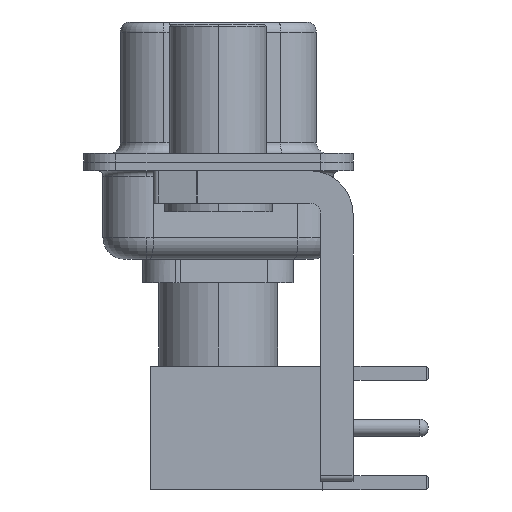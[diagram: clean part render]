
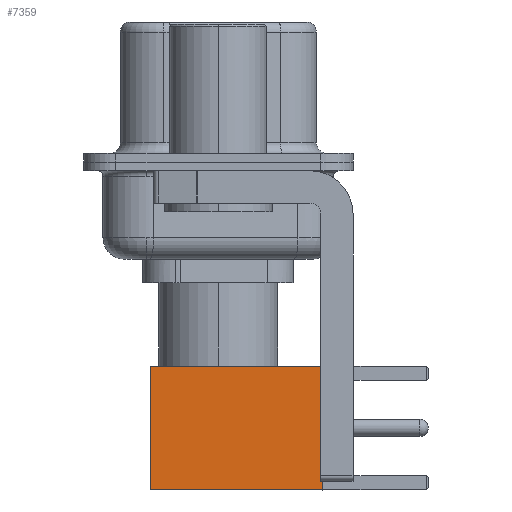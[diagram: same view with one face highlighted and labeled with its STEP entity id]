
A CAD part, left-side view. The second image highlights one B-rep face of the part: STEP entity #7359.
In plain terms, the highlighted face is planar.
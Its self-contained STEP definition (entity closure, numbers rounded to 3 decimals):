
#62 = CARTESIAN_POINT ( 'NONE',  ( 2.875, 2.875, 0. ) ) ;
#349 = CARTESIAN_POINT ( 'NONE',  ( 0., 2.875, 0. ) ) ;
#1398 = CARTESIAN_POINT ( 'NONE',  ( 2.875, 2.875, 0. ) ) ;
#1519 = PLANE ( 'NONE',  #4300 ) ;
#1608 = ORIENTED_EDGE ( 'NONE', *, *, #13072, .T. ) ;
#2622 = DIRECTION ( 'NONE',  ( -1., 0., 0. ) ) ;
#2772 = CARTESIAN_POINT ( 'NONE',  ( 2.875, 2.875, 8. ) ) ;
#3257 = EDGE_CURVE ( 'NONE', #22337, #13347, #16486, .T. ) ;
#3267 = DIRECTION ( 'NONE',  ( 0., 0., -1. ) ) ;
#3311 = DIRECTION ( 'NONE',  ( 0., 0., -1. ) ) ;
#4288 = VECTOR ( 'NONE', #19994, 1000. ) ;
#4300 = AXIS2_PLACEMENT_3D ( 'NONE', #1398, #22330, #18962 ) ;
#4686 = VECTOR ( 'NONE', #3267, 1000. ) ;
#4889 = LINE ( 'NONE', #20213, #4686 ) ;
#5431 = CARTESIAN_POINT ( 'NONE',  ( 2.875, 2.875, 0. ) ) ;
#6907 = VECTOR ( 'NONE', #3311, 1000. ) ;
#7359 = ADVANCED_FACE ( 'NONE', ( #12307 ), #1519, .T. ) ;
#8625 = LINE ( 'NONE', #14405, #22210 ) ;
#10585 = VERTEX_POINT ( 'NONE', #17837 ) ;
#10707 = EDGE_LOOP ( 'NONE', ( #22501, #1608, #11503, #21475 ) ) ;
#11503 = ORIENTED_EDGE ( 'NONE', *, *, #12285, .F. ) ;
#12285 = EDGE_CURVE ( 'NONE', #16472, #10585, #4889, .T. ) ;
#12307 = FACE_OUTER_BOUND ( 'NONE', #10707, .T. ) ;
#13072 = EDGE_CURVE ( 'NONE', #13347, #10585, #15763, .T. ) ;
#13347 = VERTEX_POINT ( 'NONE', #62 ) ;
#14405 = CARTESIAN_POINT ( 'NONE',  ( 0., 2.875, 8. ) ) ;
#15763 = LINE ( 'NONE', #349, #4288 ) ;
#16472 = VERTEX_POINT ( 'NONE', #17149 ) ;
#16486 = LINE ( 'NONE', #5431, #6907 ) ;
#17149 = CARTESIAN_POINT ( 'NONE',  ( -2.875, 2.875, 8. ) ) ;
#17837 = CARTESIAN_POINT ( 'NONE',  ( -2.875, 2.875, 0. ) ) ;
#18962 = DIRECTION ( 'NONE',  ( 0., 0., 1. ) ) ;
#19994 = DIRECTION ( 'NONE',  ( -1., 0., 0. ) ) ;
#20213 = CARTESIAN_POINT ( 'NONE',  ( -2.875, 2.875, 0. ) ) ;
#21475 = ORIENTED_EDGE ( 'NONE', *, *, #22835, .F. ) ;
#22210 = VECTOR ( 'NONE', #2622, 1000. ) ;
#22330 = DIRECTION ( 'NONE',  ( 0., 1., 0. ) ) ;
#22337 = VERTEX_POINT ( 'NONE', #2772 ) ;
#22501 = ORIENTED_EDGE ( 'NONE', *, *, #3257, .T. ) ;
#22835 = EDGE_CURVE ( 'NONE', #22337, #16472, #8625, .T. ) ;
